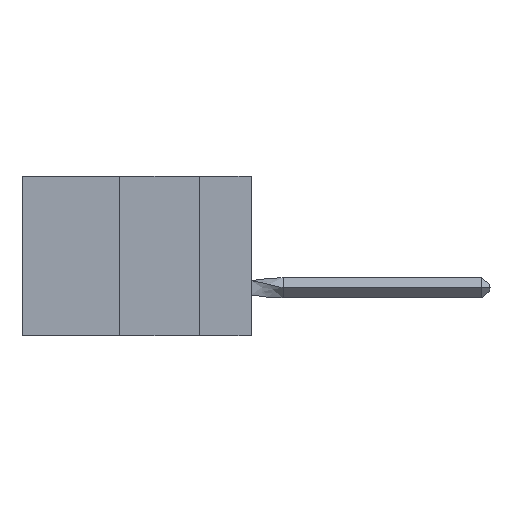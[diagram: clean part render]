
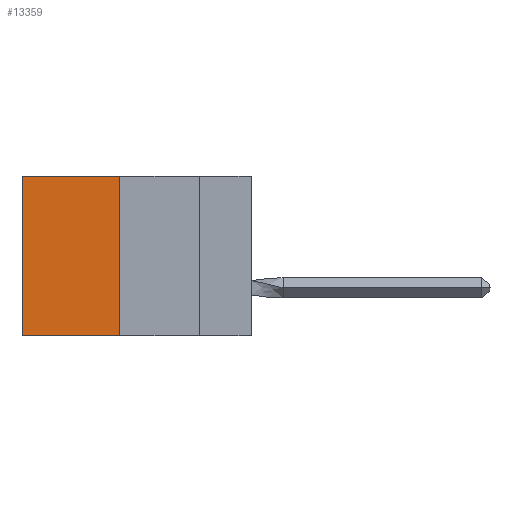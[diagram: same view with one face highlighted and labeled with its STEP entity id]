
A CAD part, left-side view. The second image highlights one B-rep face of the part: STEP entity #13359.
In plain terms, the highlighted planar face has unit normal (-1, 0, 0).
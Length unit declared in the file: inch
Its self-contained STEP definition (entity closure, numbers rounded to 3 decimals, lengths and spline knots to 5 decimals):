
#386 = CARTESIAN_POINT ( 'NONE',  ( 0.305, 0.413, -0.5 ) ) ;
#1190 = CARTESIAN_POINT ( 'NONE',  ( 0.305, 0.72, -0.5 ) ) ;
#3537 = DIRECTION ( 'NONE',  ( 0., 0., -1. ) ) ;
#3916 = LINE ( 'NONE', #8779, #6649 ) ;
#4563 = VERTEX_POINT ( 'NONE', #5964 ) ;
#5398 = ORIENTED_EDGE ( 'NONE', *, *, #6413, .T. ) ;
#5964 = CARTESIAN_POINT ( 'NONE',  ( 0.305, 0.72, 0. ) ) ;
#6347 = VECTOR ( 'NONE', #3537, 39.37008 ) ;
#6349 = VERTEX_POINT ( 'NONE', #14709 ) ;
#6413 = EDGE_CURVE ( 'NONE', #4563, #13815, #16005, .T. ) ;
#6649 = VECTOR ( 'NONE', #11240, 39.37008 ) ;
#7100 = EDGE_LOOP ( 'NONE', ( #5398, #12175, #7881, #9821 ) ) ;
#7579 = DIRECTION ( 'NONE',  ( 0., 1., 0. ) ) ;
#7881 = ORIENTED_EDGE ( 'NONE', *, *, #8070, .F. ) ;
#8070 = EDGE_CURVE ( 'NONE', #13027, #6349, #3916, .T. ) ;
#8086 = DIRECTION ( 'NONE',  ( 0., 1., 0. ) ) ;
#8179 = VECTOR ( 'NONE', #8086, 39.37008 ) ;
#8343 = EDGE_CURVE ( 'NONE', #6349, #13815, #12743, .T. ) ;
#8496 = CARTESIAN_POINT ( 'NONE',  ( 0.305, 0.72, -0.5 ) ) ;
#8614 = CARTESIAN_POINT ( 'NONE',  ( 0.305, 0.413, -0.5 ) ) ;
#8779 = CARTESIAN_POINT ( 'NONE',  ( 0.305, 0.413, -0.5 ) ) ;
#8890 = AXIS2_PLACEMENT_3D ( 'NONE', #386, #13107, #10625 ) ;
#9279 = EDGE_CURVE ( 'NONE', #13027, #4563, #14271, .T. ) ;
#9821 = ORIENTED_EDGE ( 'NONE', *, *, #9279, .T. ) ;
#10028 = FACE_OUTER_BOUND ( 'NONE', #7100, .T. ) ;
#10625 = DIRECTION ( 'NONE',  ( 0., 0., -1. ) ) ;
#11240 = DIRECTION ( 'NONE',  ( 0., 0., -1. ) ) ;
#11741 = PLANE ( 'NONE',  #8890 ) ;
#12175 = ORIENTED_EDGE ( 'NONE', *, *, #8343, .F. ) ;
#12356 = CARTESIAN_POINT ( 'NONE',  ( 0.305, 0.413, 0. ) ) ;
#12743 = LINE ( 'NONE', #8614, #14298 ) ;
#13027 = VERTEX_POINT ( 'NONE', #12356 ) ;
#13107 = DIRECTION ( 'NONE',  ( 1., 0., 0. ) ) ;
#13359 = ADVANCED_FACE ( 'NONE', ( #10028 ), #11741, .F. ) ;
#13815 = VERTEX_POINT ( 'NONE', #1190 ) ;
#14271 = LINE ( 'NONE', #15662, #8179 ) ;
#14298 = VECTOR ( 'NONE', #7579, 39.37008 ) ;
#14709 = CARTESIAN_POINT ( 'NONE',  ( 0.305, 0.413, -0.5 ) ) ;
#15662 = CARTESIAN_POINT ( 'NONE',  ( 0.305, 0.413, 0. ) ) ;
#16005 = LINE ( 'NONE', #8496, #6347 ) ;
